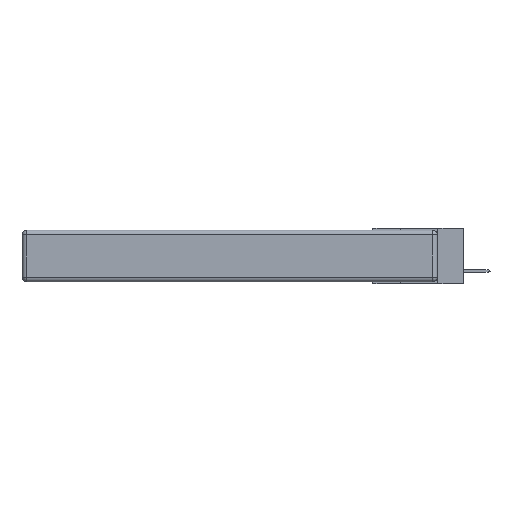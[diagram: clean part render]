
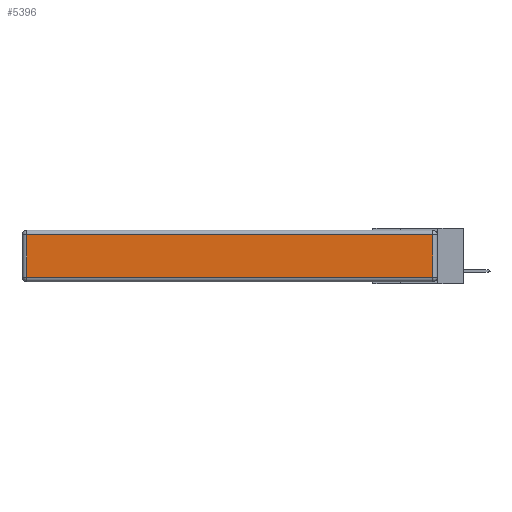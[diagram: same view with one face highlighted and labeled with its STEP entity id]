
A CAD part, left-side view. The second image highlights one B-rep face of the part: STEP entity #5396.
In plain terms, the highlighted planar face has unit normal (-1, 0, 0).
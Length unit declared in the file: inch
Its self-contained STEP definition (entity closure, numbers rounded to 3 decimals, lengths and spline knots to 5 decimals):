
#109 = DIRECTION ( 'NONE',  ( 0., -1., 0. ) ) ;
#206 = DIRECTION ( 'NONE',  ( 0., 0., 1. ) ) ;
#540 = CARTESIAN_POINT ( 'NONE',  ( 0., 0., -0.343 ) ) ;
#1139 = EDGE_CURVE ( 'NONE', #3033, #7975, #8923, .T. ) ;
#1172 = VERTEX_POINT ( 'NONE', #11931 ) ;
#1313 = CARTESIAN_POINT ( 'NONE',  ( 0., 2.72, -0.343 ) ) ;
#2069 = CARTESIAN_POINT ( 'NONE',  ( 0., 2.75, -0.03 ) ) ;
#2431 = DIRECTION ( 'NONE',  ( 0., 0., -1. ) ) ;
#2487 = CARTESIAN_POINT ( 'NONE',  ( 0., 2.72, -0.313 ) ) ;
#3033 = VERTEX_POINT ( 'NONE', #8625 ) ;
#3561 = VECTOR ( 'NONE', #206, 39.37008 ) ;
#4502 = ORIENTED_EDGE ( 'NONE', *, *, #10148, .T. ) ;
#5396 = ADVANCED_FACE ( 'NONE', ( #6315 ), #6337, .T. ) ;
#5615 = VECTOR ( 'NONE', #2431, 39.37008 ) ;
#5960 = LINE ( 'NONE', #13913, #6342 ) ;
#6227 = AXIS2_PLACEMENT_3D ( 'NONE', #540, #8744, #7517 ) ;
#6315 = FACE_OUTER_BOUND ( 'NONE', #10291, .T. ) ;
#6337 = PLANE ( 'NONE',  #6227 ) ;
#6342 = VECTOR ( 'NONE', #109, 39.37008 ) ;
#6705 = ORIENTED_EDGE ( 'NONE', *, *, #12215, .T. ) ;
#7517 = DIRECTION ( 'NONE',  ( 0., 0., 1. ) ) ;
#7749 = ORIENTED_EDGE ( 'NONE', *, *, #10008, .T. ) ;
#7975 = VERTEX_POINT ( 'NONE', #2487 ) ;
#8625 = CARTESIAN_POINT ( 'NONE',  ( 0., 2.72, -0.03 ) ) ;
#8710 = VERTEX_POINT ( 'NONE', #13191 ) ;
#8744 = DIRECTION ( 'NONE',  ( -1., 0., 0. ) ) ;
#8853 = VECTOR ( 'NONE', #11396, 39.37008 ) ;
#8923 = LINE ( 'NONE', #1313, #5615 ) ;
#9798 = CARTESIAN_POINT ( 'NONE',  ( 0., 0.03, -0.343 ) ) ;
#10008 = EDGE_CURVE ( 'NONE', #7975, #8710, #5960, .T. ) ;
#10148 = EDGE_CURVE ( 'NONE', #8710, #1172, #13864, .T. ) ;
#10291 = EDGE_LOOP ( 'NONE', ( #7749, #4502, #6705, #13563 ) ) ;
#11396 = DIRECTION ( 'NONE',  ( 0., 1., 0. ) ) ;
#11931 = CARTESIAN_POINT ( 'NONE',  ( 0., 0.03, -0.03 ) ) ;
#11980 = LINE ( 'NONE', #2069, #8853 ) ;
#12215 = EDGE_CURVE ( 'NONE', #1172, #3033, #11980, .T. ) ;
#13191 = CARTESIAN_POINT ( 'NONE',  ( 0., 0.03, -0.313 ) ) ;
#13563 = ORIENTED_EDGE ( 'NONE', *, *, #1139, .T. ) ;
#13864 = LINE ( 'NONE', #9798, #3561 ) ;
#13913 = CARTESIAN_POINT ( 'NONE',  ( 0., 0., -0.313 ) ) ;
